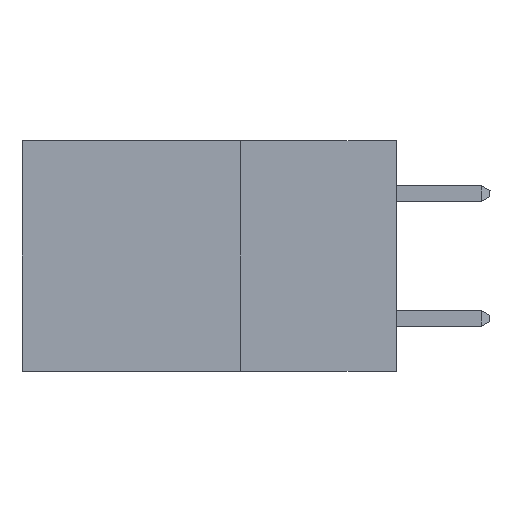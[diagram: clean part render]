
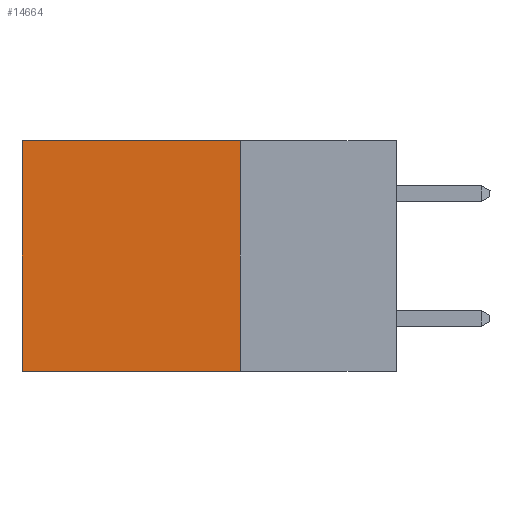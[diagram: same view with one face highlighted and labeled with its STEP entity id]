
A CAD part, left-side view. The second image highlights one B-rep face of the part: STEP entity #14664.
In plain terms, the highlighted planar face has unit normal (-1, 0, 0).
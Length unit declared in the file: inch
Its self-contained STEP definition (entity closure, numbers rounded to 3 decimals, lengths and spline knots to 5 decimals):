
#142 = EDGE_CURVE ( 'NONE', #12595, #3755, #14654, .T. ) ;
#680 = DIRECTION ( 'NONE',  ( 0., 0., -1. ) ) ;
#959 = LINE ( 'NONE', #11566, #9884 ) ;
#2828 = CARTESIAN_POINT ( 'NONE',  ( 0.298, 0.6, 0. ) ) ;
#3126 = LINE ( 'NONE', #11040, #5816 ) ;
#3755 = VERTEX_POINT ( 'NONE', #14663 ) ;
#3847 = EDGE_LOOP ( 'NONE', ( #11184, #13393, #5454, #7732 ) ) ;
#3945 = DIRECTION ( 'NONE',  ( 1., 0., 0. ) ) ;
#4220 = LINE ( 'NONE', #7472, #12965 ) ;
#4228 = CARTESIAN_POINT ( 'NONE',  ( 0.298, 0.25, -0.37 ) ) ;
#5454 = ORIENTED_EDGE ( 'NONE', *, *, #6130, .F. ) ;
#5578 = VECTOR ( 'NONE', #680, 39.37008 ) ;
#5816 = VECTOR ( 'NONE', #6493, 39.37008 ) ;
#6130 = EDGE_CURVE ( 'NONE', #9673, #8253, #4220, .T. ) ;
#6264 = CARTESIAN_POINT ( 'NONE',  ( 0.298, 0.25, 0. ) ) ;
#6269 = AXIS2_PLACEMENT_3D ( 'NONE', #9580, #3945, #11882 ) ;
#6493 = DIRECTION ( 'NONE',  ( 0., 1., 0. ) ) ;
#7472 = CARTESIAN_POINT ( 'NONE',  ( 0.298, 0.25, 0. ) ) ;
#7732 = ORIENTED_EDGE ( 'NONE', *, *, #11871, .T. ) ;
#8253 = VERTEX_POINT ( 'NONE', #4228 ) ;
#8611 = DIRECTION ( 'NONE',  ( 0., 0., -1. ) ) ;
#9580 = CARTESIAN_POINT ( 'NONE',  ( 0.298, 0.25, 0. ) ) ;
#9673 = VERTEX_POINT ( 'NONE', #6264 ) ;
#9884 = VECTOR ( 'NONE', #11614, 39.37008 ) ;
#11040 = CARTESIAN_POINT ( 'NONE',  ( 0.298, 0.25, 0. ) ) ;
#11184 = ORIENTED_EDGE ( 'NONE', *, *, #142, .T. ) ;
#11468 = CARTESIAN_POINT ( 'NONE',  ( 0.298, 0.6, 0. ) ) ;
#11566 = CARTESIAN_POINT ( 'NONE',  ( 0.298, 0.25, -0.37 ) ) ;
#11614 = DIRECTION ( 'NONE',  ( 0., 1., 0. ) ) ;
#11871 = EDGE_CURVE ( 'NONE', #9673, #12595, #3126, .T. ) ;
#11882 = DIRECTION ( 'NONE',  ( 0., 0., -1. ) ) ;
#12595 = VERTEX_POINT ( 'NONE', #11468 ) ;
#12965 = VECTOR ( 'NONE', #8611, 39.37008 ) ;
#13393 = ORIENTED_EDGE ( 'NONE', *, *, #14518, .F. ) ;
#13825 = FACE_OUTER_BOUND ( 'NONE', #3847, .T. ) ;
#14128 = PLANE ( 'NONE',  #6269 ) ;
#14518 = EDGE_CURVE ( 'NONE', #8253, #3755, #959, .T. ) ;
#14654 = LINE ( 'NONE', #2828, #5578 ) ;
#14663 = CARTESIAN_POINT ( 'NONE',  ( 0.298, 0.6, -0.37 ) ) ;
#14664 = ADVANCED_FACE ( 'NONE', ( #13825 ), #14128, .F. ) ;
